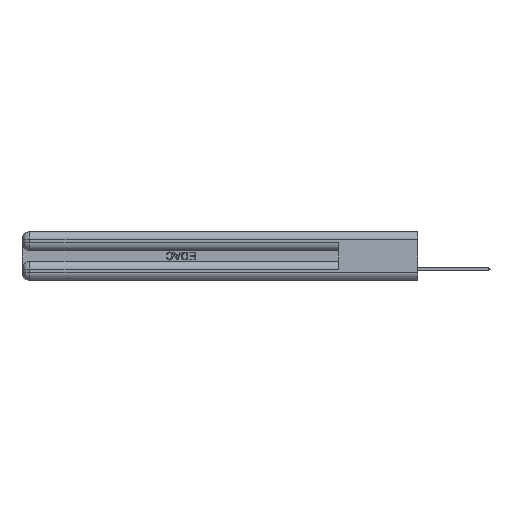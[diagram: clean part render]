
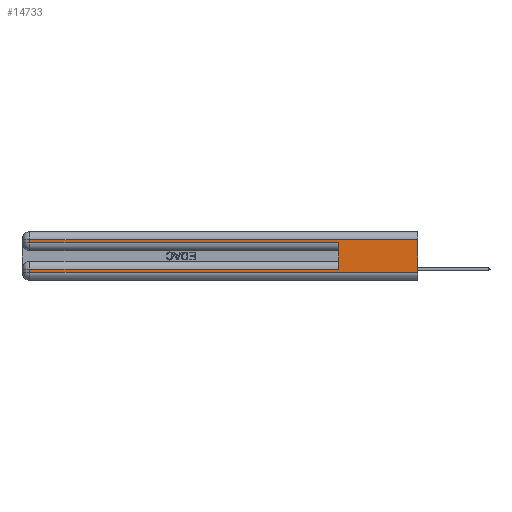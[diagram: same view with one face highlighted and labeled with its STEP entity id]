
A CAD part, left-side view. The second image highlights one B-rep face of the part: STEP entity #14733.
In plain terms, the highlighted planar face has unit normal (-1, 0, 0).
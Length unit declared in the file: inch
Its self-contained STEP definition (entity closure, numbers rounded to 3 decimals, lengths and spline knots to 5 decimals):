
#12 = ORIENTED_EDGE ( 'NONE', *, *, #7816, .T. ) ;
#599 = ORIENTED_EDGE ( 'NONE', *, *, #34733, .T. ) ;
#813 = CARTESIAN_POINT ( 'NONE',  ( 0., 2.94, 0.285 ) ) ;
#1019 = LINE ( 'NONE', #15912, #34854 ) ;
#1478 = CARTESIAN_POINT ( 'NONE',  ( 0., 0., 0.06 ) ) ;
#2381 = VECTOR ( 'NONE', #19542, 39.37008 ) ;
#4040 = VECTOR ( 'NONE', #12930, 39.37008 ) ;
#4443 = VERTEX_POINT ( 'NONE', #36614 ) ;
#4635 = EDGE_CURVE ( 'NONE', #20013, #25935, #38625, .T. ) ;
#6514 = DIRECTION ( 'NONE',  ( 0., -1., 0. ) ) ;
#6708 = CARTESIAN_POINT ( 'NONE',  ( 0., 0., 0.085 ) ) ;
#7234 = LINE ( 'NONE', #6708, #22573 ) ;
#7242 = VERTEX_POINT ( 'NONE', #36080 ) ;
#7474 = ORIENTED_EDGE ( 'NONE', *, *, #4635, .T. ) ;
#7753 = VERTEX_POINT ( 'NONE', #32028 ) ;
#7816 = EDGE_CURVE ( 'NONE', #25935, #32434, #32031, .T. ) ;
#10393 = VECTOR ( 'NONE', #6514, 39.37008 ) ;
#10435 = DIRECTION ( 'NONE',  ( 0., 1., 0. ) ) ;
#12654 = ORIENTED_EDGE ( 'NONE', *, *, #17623, .F. ) ;
#12930 = DIRECTION ( 'NONE',  ( 0., 0., -1. ) ) ;
#12958 = DIRECTION ( 'NONE',  ( 0., -1., 0. ) ) ;
#13842 = CARTESIAN_POINT ( 'NONE',  ( 0., 2.94, 0.31 ) ) ;
#13906 = VECTOR ( 'NONE', #12958, 39.37008 ) ;
#14387 = EDGE_CURVE ( 'NONE', #4443, #38988, #43606, .T. ) ;
#14408 = ORIENTED_EDGE ( 'NONE', *, *, #22605, .F. ) ;
#14453 = FACE_OUTER_BOUND ( 'NONE', #41354, .T. ) ;
#14733 = ADVANCED_FACE ( 'NONE', ( #14453 ), #18743, .F. ) ;
#15912 = CARTESIAN_POINT ( 'NONE',  ( 0., 0., 0.31 ) ) ;
#17549 = DIRECTION ( 'NONE',  ( 0., 1., 0. ) ) ;
#17623 = EDGE_CURVE ( 'NONE', #19848, #38988, #38959, .T. ) ;
#18127 = EDGE_CURVE ( 'NONE', #19848, #20013, #1019, .T. ) ;
#18743 = PLANE ( 'NONE',  #23622 ) ;
#19358 = DIRECTION ( 'NONE',  ( 1., 0., 0. ) ) ;
#19542 = DIRECTION ( 'NONE',  ( 0., 0., -1. ) ) ;
#19848 = VERTEX_POINT ( 'NONE', #38721 ) ;
#19999 = DIRECTION ( 'NONE',  ( 0., 0., -1. ) ) ;
#20013 = VERTEX_POINT ( 'NONE', #13842 ) ;
#20719 = CARTESIAN_POINT ( 'NONE',  ( 0., 0., 0.285 ) ) ;
#22573 = VECTOR ( 'NONE', #10435, 39.37008 ) ;
#22605 = EDGE_CURVE ( 'NONE', #7753, #32434, #30986, .T. ) ;
#23622 = AXIS2_PLACEMENT_3D ( 'NONE', #37564, #19358, #34050 ) ;
#25935 = VERTEX_POINT ( 'NONE', #813 ) ;
#27246 = CARTESIAN_POINT ( 'NONE',  ( 0., 0., 0.06 ) ) ;
#30986 = LINE ( 'NONE', #41055, #43628 ) ;
#31011 = CARTESIAN_POINT ( 'NONE',  ( 0., 2.94, 0.37 ) ) ;
#32028 = CARTESIAN_POINT ( 'NONE',  ( 0., 0.6, 0.085 ) ) ;
#32031 = LINE ( 'NONE', #20719, #10393 ) ;
#32434 = VERTEX_POINT ( 'NONE', #33947 ) ;
#33947 = CARTESIAN_POINT ( 'NONE',  ( 0., 0.6, 0.285 ) ) ;
#34050 = DIRECTION ( 'NONE',  ( 0., 0., -1. ) ) ;
#34733 = EDGE_CURVE ( 'NONE', #7753, #7242, #7234, .T. ) ;
#34768 = CARTESIAN_POINT ( 'NONE',  ( 0., 0., 0.37 ) ) ;
#34854 = VECTOR ( 'NONE', #17549, 39.37008 ) ;
#34932 = ORIENTED_EDGE ( 'NONE', *, *, #14387, .T. ) ;
#35212 = VECTOR ( 'NONE', #19999, 39.37008 ) ;
#36080 = CARTESIAN_POINT ( 'NONE',  ( 0., 2.94, 0.085 ) ) ;
#36614 = CARTESIAN_POINT ( 'NONE',  ( 0., 2.94, 0.06 ) ) ;
#37378 = ORIENTED_EDGE ( 'NONE', *, *, #46258, .T. ) ;
#37564 = CARTESIAN_POINT ( 'NONE',  ( 0., 0., 0.37 ) ) ;
#38625 = LINE ( 'NONE', #31011, #35212 ) ;
#38721 = CARTESIAN_POINT ( 'NONE',  ( 0., 0., 0.31 ) ) ;
#38959 = LINE ( 'NONE', #34768, #4040 ) ;
#38988 = VERTEX_POINT ( 'NONE', #1478 ) ;
#40692 = LINE ( 'NONE', #41436, #2381 ) ;
#41055 = CARTESIAN_POINT ( 'NONE',  ( 0., 0.6, 0.145 ) ) ;
#41354 = EDGE_LOOP ( 'NONE', ( #12654, #43800, #7474, #12, #14408, #599, #37378, #34932 ) ) ;
#41436 = CARTESIAN_POINT ( 'NONE',  ( 0., 2.94, 0.37 ) ) ;
#43606 = LINE ( 'NONE', #27246, #13906 ) ;
#43628 = VECTOR ( 'NONE', #44749, 39.37008 ) ;
#43800 = ORIENTED_EDGE ( 'NONE', *, *, #18127, .T. ) ;
#44749 = DIRECTION ( 'NONE',  ( 0., 0., 1. ) ) ;
#46258 = EDGE_CURVE ( 'NONE', #7242, #4443, #40692, .T. ) ;
